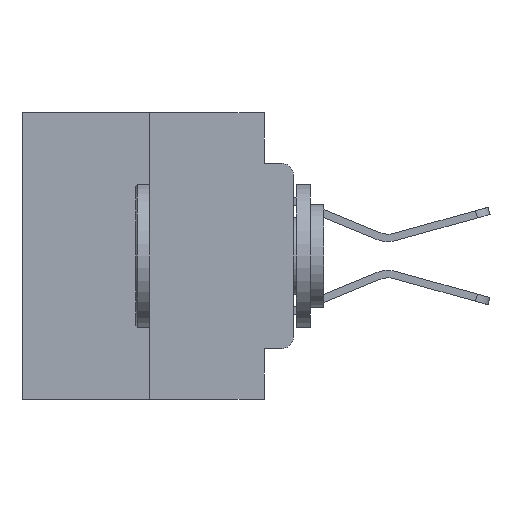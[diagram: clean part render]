
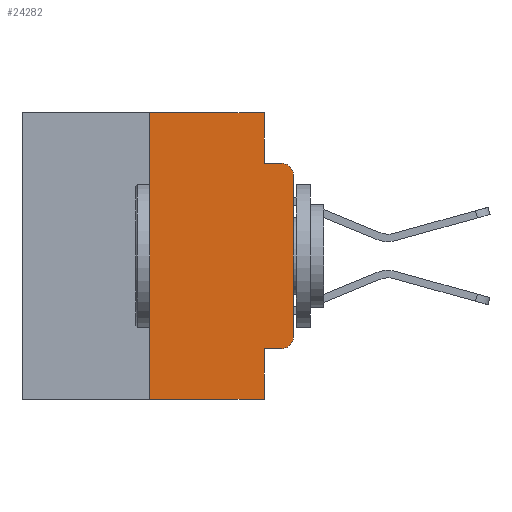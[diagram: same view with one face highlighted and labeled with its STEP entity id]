
A CAD part, left-side view. The second image highlights one B-rep face of the part: STEP entity #24282.
In plain terms, the highlighted planar face has unit normal (-1, 0, 0).
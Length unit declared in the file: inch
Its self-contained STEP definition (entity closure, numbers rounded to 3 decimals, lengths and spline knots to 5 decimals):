
#476 = LINE ( 'NONE', #19619, #18317 ) ;
#655 = CIRCLE ( 'NONE', #3857, 0.02 ) ;
#723 = EDGE_CURVE ( 'NONE', #17675, #4921, #17918, .T. ) ;
#918 = VECTOR ( 'NONE', #5154, 39.37008 ) ;
#1420 = CARTESIAN_POINT ( 'NONE',  ( 0., 0.02, -0.1085 ) ) ;
#2037 = LINE ( 'NONE', #23651, #19804 ) ;
#2425 = ORIENTED_EDGE ( 'NONE', *, *, #12981, .T. ) ;
#2995 = CARTESIAN_POINT ( 'NONE',  ( 0., 0.25, 0. ) ) ;
#3383 = LINE ( 'NONE', #3531, #26800 ) ;
#3504 = ORIENTED_EDGE ( 'NONE', *, *, #11619, .T. ) ;
#3531 = CARTESIAN_POINT ( 'NONE',  ( 0., 0.473, 0. ) ) ;
#3857 = AXIS2_PLACEMENT_3D ( 'NONE', #5729, #20488, #8000 ) ;
#4123 = CARTESIAN_POINT ( 'NONE',  ( 0., 0.051, 0. ) ) ;
#4410 = VERTEX_POINT ( 'NONE', #25008 ) ;
#4884 = DIRECTION ( 'NONE',  ( 0., 0., -1. ) ) ;
#4921 = VERTEX_POINT ( 'NONE', #25560 ) ;
#5137 = DIRECTION ( 'NONE',  ( 0., -1., 0. ) ) ;
#5154 = DIRECTION ( 'NONE',  ( 0., -1., 0. ) ) ;
#5251 = EDGE_CURVE ( 'NONE', #4410, #11434, #655, .T. ) ;
#5312 = CARTESIAN_POINT ( 'NONE',  ( 0., 0., -0.3915 ) ) ;
#5519 = ORIENTED_EDGE ( 'NONE', *, *, #15307, .F. ) ;
#5729 = CARTESIAN_POINT ( 'NONE',  ( 0., 0.02, -0.3915 ) ) ;
#5922 = EDGE_CURVE ( 'NONE', #17675, #16354, #12460, .T. ) ;
#6049 = ORIENTED_EDGE ( 'NONE', *, *, #5251, .T. ) ;
#7257 = PLANE ( 'NONE',  #26888 ) ;
#7920 = VERTEX_POINT ( 'NONE', #12298 ) ;
#8000 = DIRECTION ( 'NONE',  ( 0., 0., -1. ) ) ;
#8317 = VERTEX_POINT ( 'NONE', #13263 ) ;
#8566 = ORIENTED_EDGE ( 'NONE', *, *, #12019, .F. ) ;
#8687 = VERTEX_POINT ( 'NONE', #11648 ) ;
#9382 = ORIENTED_EDGE ( 'NONE', *, *, #723, .T. ) ;
#9809 = LINE ( 'NONE', #24404, #918 ) ;
#11048 = CARTESIAN_POINT ( 'NONE',  ( 0., 0.051, -0.4115 ) ) ;
#11207 = VECTOR ( 'NONE', #21222, 39.37008 ) ;
#11414 = ORIENTED_EDGE ( 'NONE', *, *, #26176, .F. ) ;
#11434 = VERTEX_POINT ( 'NONE', #5312 ) ;
#11473 = DIRECTION ( 'NONE',  ( 1., 0., 0. ) ) ;
#11619 = EDGE_CURVE ( 'NONE', #11434, #8317, #476, .T. ) ;
#11648 = CARTESIAN_POINT ( 'NONE',  ( 0., 0.051, -0.4115 ) ) ;
#11933 = VERTEX_POINT ( 'NONE', #16158 ) ;
#12019 = EDGE_CURVE ( 'NONE', #16354, #11933, #3383, .T. ) ;
#12298 = CARTESIAN_POINT ( 'NONE',  ( 0., 0.02, -0.0885 ) ) ;
#12460 = LINE ( 'NONE', #15100, #22690 ) ;
#12711 = AXIS2_PLACEMENT_3D ( 'NONE', #1420, #16021, #14207 ) ;
#12981 = EDGE_CURVE ( 'NONE', #8317, #7920, #14948, .T. ) ;
#13263 = CARTESIAN_POINT ( 'NONE',  ( 0., 0., -0.1085 ) ) ;
#13717 = FACE_OUTER_BOUND ( 'NONE', #21791, .T. ) ;
#14207 = DIRECTION ( 'NONE',  ( 0., 0., -1. ) ) ;
#14308 = DIRECTION ( 'NONE',  ( 0., -1., 0. ) ) ;
#14948 = CIRCLE ( 'NONE', #12711, 0.02 ) ;
#15100 = CARTESIAN_POINT ( 'NONE',  ( 0., 0.25, 0. ) ) ;
#15228 = ORIENTED_EDGE ( 'NONE', *, *, #17643, .T. ) ;
#15307 = EDGE_CURVE ( 'NONE', #11933, #27231, #23336, .T. ) ;
#15522 = CARTESIAN_POINT ( 'NONE',  ( 0., 0.25, -0.5 ) ) ;
#16021 = DIRECTION ( 'NONE',  ( -1., 0., 0. ) ) ;
#16158 = CARTESIAN_POINT ( 'NONE',  ( 0., 0.051, 0. ) ) ;
#16354 = VERTEX_POINT ( 'NONE', #2995 ) ;
#16492 = VECTOR ( 'NONE', #5137, 39.37008 ) ;
#17080 = DIRECTION ( 'NONE',  ( 0., 0., 1. ) ) ;
#17294 = ORIENTED_EDGE ( 'NONE', *, *, #5922, .F. ) ;
#17643 = EDGE_CURVE ( 'NONE', #8687, #4410, #19885, .T. ) ;
#17675 = VERTEX_POINT ( 'NONE', #15522 ) ;
#17874 = EDGE_CURVE ( 'NONE', #8687, #4921, #2037, .T. ) ;
#17918 = LINE ( 'NONE', #26214, #16492 ) ;
#18317 = VECTOR ( 'NONE', #19899, 39.37008 ) ;
#19607 = DIRECTION ( 'NONE',  ( 0., -1., 0. ) ) ;
#19619 = CARTESIAN_POINT ( 'NONE',  ( 0., 0., 0. ) ) ;
#19804 = VECTOR ( 'NONE', #23516, 39.37008 ) ;
#19885 = LINE ( 'NONE', #11048, #24293 ) ;
#19899 = DIRECTION ( 'NONE',  ( 0., 0., 1. ) ) ;
#20488 = DIRECTION ( 'NONE',  ( -1., 0., 0. ) ) ;
#21222 = DIRECTION ( 'NONE',  ( 0., 0., -1. ) ) ;
#21791 = EDGE_LOOP ( 'NONE', ( #3504, #2425, #11414, #5519, #8566, #17294, #9382, #24821, #15228, #6049 ) ) ;
#22690 = VECTOR ( 'NONE', #17080, 39.37008 ) ;
#23336 = LINE ( 'NONE', #4123, #11207 ) ;
#23516 = DIRECTION ( 'NONE',  ( 0., 0., -1. ) ) ;
#23651 = CARTESIAN_POINT ( 'NONE',  ( 0., 0.051, 0. ) ) ;
#24121 = CARTESIAN_POINT ( 'NONE',  ( 0., 0.473, 0. ) ) ;
#24282 = ADVANCED_FACE ( 'NONE', ( #13717 ), #7257, .F. ) ;
#24293 = VECTOR ( 'NONE', #19607, 39.37008 ) ;
#24404 = CARTESIAN_POINT ( 'NONE',  ( 0., 0.051, -0.0885 ) ) ;
#24821 = ORIENTED_EDGE ( 'NONE', *, *, #17874, .F. ) ;
#25008 = CARTESIAN_POINT ( 'NONE',  ( 0., 0.02, -0.4115 ) ) ;
#25231 = CARTESIAN_POINT ( 'NONE',  ( 0., 0.051, -0.0885 ) ) ;
#25560 = CARTESIAN_POINT ( 'NONE',  ( 0., 0.051, -0.5 ) ) ;
#26176 = EDGE_CURVE ( 'NONE', #27231, #7920, #9809, .T. ) ;
#26214 = CARTESIAN_POINT ( 'NONE',  ( 0., 0.473, -0.5 ) ) ;
#26800 = VECTOR ( 'NONE', #14308, 39.37008 ) ;
#26888 = AXIS2_PLACEMENT_3D ( 'NONE', #24121, #11473, #4884 ) ;
#27231 = VERTEX_POINT ( 'NONE', #25231 ) ;
